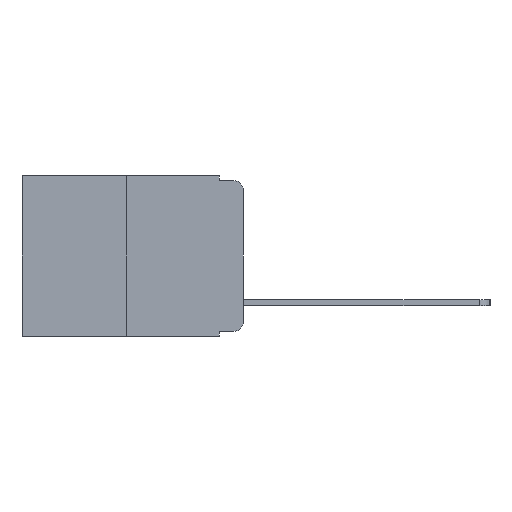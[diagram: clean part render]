
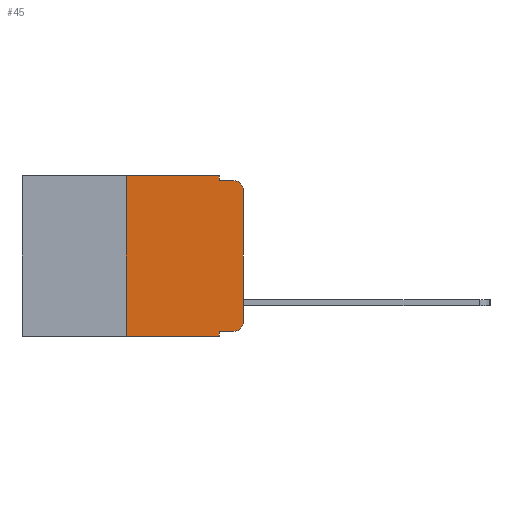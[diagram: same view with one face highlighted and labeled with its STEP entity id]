
A CAD part, left-side view. The second image highlights one B-rep face of the part: STEP entity #45.
In plain terms, the highlighted planar face has unit normal (-1, 0, 0).
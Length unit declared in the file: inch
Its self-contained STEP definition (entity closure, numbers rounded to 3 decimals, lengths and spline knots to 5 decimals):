
#45 = ADVANCED_FACE ( 'NONE', ( #10217 ), #2141, .F. ) ;
#337 = EDGE_CURVE ( 'NONE', #1273, #4715, #4541, .T. ) ;
#362 = EDGE_CURVE ( 'NONE', #9220, #2306, #3987, .T. ) ;
#425 = CARTESIAN_POINT ( 'NONE',  ( 0., 0.02, -0.333 ) ) ;
#611 = VECTOR ( 'NONE', #9125, 39.37008 ) ;
#642 = CARTESIAN_POINT ( 'NONE',  ( 0., 0.25, 0. ) ) ;
#858 = CARTESIAN_POINT ( 'NONE',  ( 0., 0.051, 0. ) ) ;
#919 = ORIENTED_EDGE ( 'NONE', *, *, #6803, .F. ) ;
#923 = AXIS2_PLACEMENT_3D ( 'NONE', #10283, #5520, #11088 ) ;
#1273 = VERTEX_POINT ( 'NONE', #3776 ) ;
#1306 = VERTEX_POINT ( 'NONE', #7417 ) ;
#1425 = VERTEX_POINT ( 'NONE', #11496 ) ;
#1488 = VERTEX_POINT ( 'NONE', #10315 ) ;
#1659 = LINE ( 'NONE', #1780, #4039 ) ;
#1765 = ORIENTED_EDGE ( 'NONE', *, *, #362, .T. ) ;
#1780 = CARTESIAN_POINT ( 'NONE',  ( 0., 0., 0. ) ) ;
#1955 = DIRECTION ( 'NONE',  ( 0., 0., 1. ) ) ;
#2141 = PLANE ( 'NONE',  #6356 ) ;
#2306 = VERTEX_POINT ( 'NONE', #2951 ) ;
#2951 = CARTESIAN_POINT ( 'NONE',  ( 0., 0., -0.313 ) ) ;
#3184 = VECTOR ( 'NONE', #5429, 39.37008 ) ;
#3248 = VERTEX_POINT ( 'NONE', #11081 ) ;
#3419 = ORIENTED_EDGE ( 'NONE', *, *, #10490, .F. ) ;
#3617 = LINE ( 'NONE', #8314, #611 ) ;
#3620 = AXIS2_PLACEMENT_3D ( 'NONE', #9172, #7593, #5398 ) ;
#3695 = CARTESIAN_POINT ( 'NONE',  ( 0., 0.473, 0. ) ) ;
#3746 = DIRECTION ( 'NONE',  ( 0., -1., 0. ) ) ;
#3776 = CARTESIAN_POINT ( 'NONE',  ( 0., 0.051, -0.333 ) ) ;
#3987 = CIRCLE ( 'NONE', #3620, 0.02 ) ;
#4039 = VECTOR ( 'NONE', #8767, 39.37008 ) ;
#4304 = CIRCLE ( 'NONE', #923, 0.02 ) ;
#4541 = LINE ( 'NONE', #858, #8619 ) ;
#4595 = VECTOR ( 'NONE', #10255, 39.37008 ) ;
#4715 = VERTEX_POINT ( 'NONE', #7957 ) ;
#4871 = DIRECTION ( 'NONE',  ( 0., 0., -1. ) ) ;
#5091 = VERTEX_POINT ( 'NONE', #8189 ) ;
#5112 = CARTESIAN_POINT ( 'NONE',  ( 0., 0.473, 0. ) ) ;
#5270 = DIRECTION ( 'NONE',  ( 0., 0., -1. ) ) ;
#5282 = DIRECTION ( 'NONE',  ( 1., 0., 0. ) ) ;
#5398 = DIRECTION ( 'NONE',  ( 0., 0., -1. ) ) ;
#5429 = DIRECTION ( 'NONE',  ( 0., -1., 0. ) ) ;
#5520 = DIRECTION ( 'NONE',  ( -1., 0., 0. ) ) ;
#5628 = LINE ( 'NONE', #642, #9606 ) ;
#5964 = VERTEX_POINT ( 'NONE', #11147 ) ;
#6334 = CARTESIAN_POINT ( 'NONE',  ( 0., 0.051, -0.333 ) ) ;
#6356 = AXIS2_PLACEMENT_3D ( 'NONE', #5112, #5282, #5270 ) ;
#6687 = EDGE_LOOP ( 'NONE', ( #11281, #10523, #919, #8959, #8604, #3419, #9819, #8496, #9364, #1765 ) ) ;
#6773 = EDGE_CURVE ( 'NONE', #1306, #3248, #11515, .T. ) ;
#6803 = EDGE_CURVE ( 'NONE', #3248, #1425, #10992, .T. ) ;
#6835 = EDGE_CURVE ( 'NONE', #1273, #9220, #8920, .T. ) ;
#6840 = VECTOR ( 'NONE', #3746, 39.37008 ) ;
#6861 = EDGE_CURVE ( 'NONE', #1488, #1425, #4304, .T. ) ;
#6897 = EDGE_CURVE ( 'NONE', #2306, #1488, #1659, .T. ) ;
#7417 = CARTESIAN_POINT ( 'NONE',  ( 0., 0.051, 0. ) ) ;
#7593 = DIRECTION ( 'NONE',  ( -1., 0., 0. ) ) ;
#7907 = CARTESIAN_POINT ( 'NONE',  ( 0., 0.051, -0.01 ) ) ;
#7957 = CARTESIAN_POINT ( 'NONE',  ( 0., 0.051, -0.343 ) ) ;
#8189 = CARTESIAN_POINT ( 'NONE',  ( 0., 0.25, -0.343 ) ) ;
#8314 = CARTESIAN_POINT ( 'NONE',  ( 0., 0.473, -0.343 ) ) ;
#8494 = EDGE_CURVE ( 'NONE', #5964, #1306, #9750, .T. ) ;
#8496 = ORIENTED_EDGE ( 'NONE', *, *, #337, .F. ) ;
#8604 = ORIENTED_EDGE ( 'NONE', *, *, #8494, .F. ) ;
#8619 = VECTOR ( 'NONE', #4871, 39.37008 ) ;
#8664 = CARTESIAN_POINT ( 'NONE',  ( 0., 0.051, 0. ) ) ;
#8767 = DIRECTION ( 'NONE',  ( 0., 0., 1. ) ) ;
#8920 = LINE ( 'NONE', #6334, #4595 ) ;
#8959 = ORIENTED_EDGE ( 'NONE', *, *, #6773, .F. ) ;
#9125 = DIRECTION ( 'NONE',  ( 0., -1., 0. ) ) ;
#9172 = CARTESIAN_POINT ( 'NONE',  ( 0., 0.02, -0.313 ) ) ;
#9220 = VERTEX_POINT ( 'NONE', #425 ) ;
#9364 = ORIENTED_EDGE ( 'NONE', *, *, #6835, .T. ) ;
#9445 = DIRECTION ( 'NONE',  ( 0., 0., -1. ) ) ;
#9606 = VECTOR ( 'NONE', #1955, 39.37008 ) ;
#9730 = EDGE_CURVE ( 'NONE', #5091, #4715, #3617, .T. ) ;
#9750 = LINE ( 'NONE', #3695, #3184 ) ;
#9819 = ORIENTED_EDGE ( 'NONE', *, *, #9730, .T. ) ;
#10217 = FACE_OUTER_BOUND ( 'NONE', #6687, .T. ) ;
#10255 = DIRECTION ( 'NONE',  ( 0., -1., 0. ) ) ;
#10283 = CARTESIAN_POINT ( 'NONE',  ( 0., 0.02, -0.03 ) ) ;
#10315 = CARTESIAN_POINT ( 'NONE',  ( 0., 0., -0.03 ) ) ;
#10490 = EDGE_CURVE ( 'NONE', #5091, #5964, #5628, .T. ) ;
#10523 = ORIENTED_EDGE ( 'NONE', *, *, #6861, .T. ) ;
#10992 = LINE ( 'NONE', #7907, #6840 ) ;
#11081 = CARTESIAN_POINT ( 'NONE',  ( 0., 0.051, -0.01 ) ) ;
#11088 = DIRECTION ( 'NONE',  ( 0., 0., -1. ) ) ;
#11147 = CARTESIAN_POINT ( 'NONE',  ( 0., 0.25, 0. ) ) ;
#11258 = VECTOR ( 'NONE', #9445, 39.37008 ) ;
#11281 = ORIENTED_EDGE ( 'NONE', *, *, #6897, .T. ) ;
#11496 = CARTESIAN_POINT ( 'NONE',  ( 0., 0.02, -0.01 ) ) ;
#11515 = LINE ( 'NONE', #8664, #11258 ) ;
